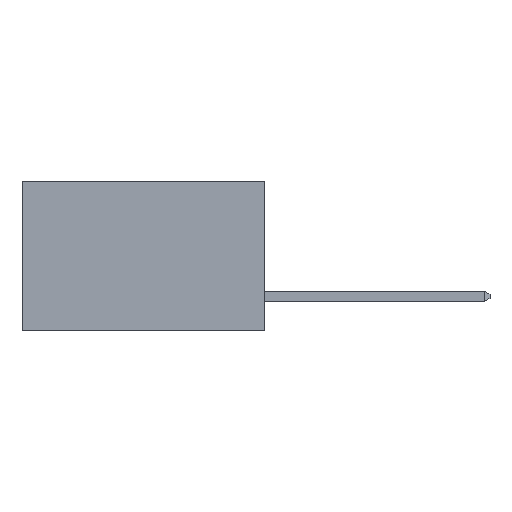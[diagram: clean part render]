
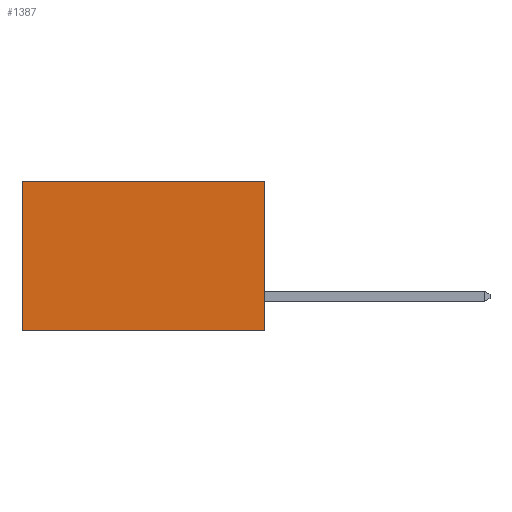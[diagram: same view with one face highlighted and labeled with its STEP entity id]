
A CAD part, left-side view. The second image highlights one B-rep face of the part: STEP entity #1387.
In plain terms, the highlighted planar face has unit normal (-1, 0, 0).
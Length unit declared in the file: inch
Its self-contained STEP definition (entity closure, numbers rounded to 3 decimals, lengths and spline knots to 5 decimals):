
#158 = VERTEX_POINT ( 'NONE', #6100 ) ;
#322 = EDGE_CURVE ( 'NONE', #1749, #3435, #7476, .T. ) ;
#447 = CARTESIAN_POINT ( 'NONE',  ( 0.2615, 0., 0. ) ) ;
#609 = DIRECTION ( 'NONE',  ( 0., 0., -1. ) ) ;
#1137 = VECTOR ( 'NONE', #8581, 39.37008 ) ;
#1387 = ADVANCED_FACE ( 'NONE', ( #3608 ), #4067, .F. ) ;
#1579 = EDGE_CURVE ( 'NONE', #158, #5817, #5837, .T. ) ;
#1749 = VERTEX_POINT ( 'NONE', #447 ) ;
#2723 = LINE ( 'NONE', #9731, #5181 ) ;
#3435 = VERTEX_POINT ( 'NONE', #5038 ) ;
#3608 = FACE_OUTER_BOUND ( 'NONE', #4856, .T. ) ;
#4022 = CARTESIAN_POINT ( 'NONE',  ( 0.2615, 0., 0. ) ) ;
#4067 = PLANE ( 'NONE',  #5044 ) ;
#4185 = ORIENTED_EDGE ( 'NONE', *, *, #1579, .F. ) ;
#4652 = LINE ( 'NONE', #5059, #7953 ) ;
#4720 = EDGE_CURVE ( 'NONE', #1749, #158, #2723, .T. ) ;
#4856 = EDGE_LOOP ( 'NONE', ( #6600, #4185, #8238, #8436 ) ) ;
#5038 = CARTESIAN_POINT ( 'NONE',  ( 0.2615, 0.6, 0. ) ) ;
#5044 = AXIS2_PLACEMENT_3D ( 'NONE', #8011, #8101, #8161 ) ;
#5059 = CARTESIAN_POINT ( 'NONE',  ( 0.2615, 0.6, -0.37 ) ) ;
#5181 = VECTOR ( 'NONE', #9720, 39.37008 ) ;
#5282 = CARTESIAN_POINT ( 'NONE',  ( 0.2615, 0.6, -0.37 ) ) ;
#5381 = VECTOR ( 'NONE', #9350, 39.37008 ) ;
#5817 = VERTEX_POINT ( 'NONE', #5282 ) ;
#5837 = LINE ( 'NONE', #9331, #5381 ) ;
#6100 = CARTESIAN_POINT ( 'NONE',  ( 0.2615, 0., -0.37 ) ) ;
#6600 = ORIENTED_EDGE ( 'NONE', *, *, #8048, .T. ) ;
#7476 = LINE ( 'NONE', #4022, #1137 ) ;
#7953 = VECTOR ( 'NONE', #609, 39.37008 ) ;
#8011 = CARTESIAN_POINT ( 'NONE',  ( 0.2615, 0., -0.37 ) ) ;
#8048 = EDGE_CURVE ( 'NONE', #3435, #5817, #4652, .T. ) ;
#8101 = DIRECTION ( 'NONE',  ( 1., 0., 0. ) ) ;
#8161 = DIRECTION ( 'NONE',  ( 0., 0., -1. ) ) ;
#8238 = ORIENTED_EDGE ( 'NONE', *, *, #4720, .F. ) ;
#8436 = ORIENTED_EDGE ( 'NONE', *, *, #322, .T. ) ;
#8581 = DIRECTION ( 'NONE',  ( 0., 1., 0. ) ) ;
#9331 = CARTESIAN_POINT ( 'NONE',  ( 0.2615, 0., -0.37 ) ) ;
#9350 = DIRECTION ( 'NONE',  ( 0., 1., 0. ) ) ;
#9720 = DIRECTION ( 'NONE',  ( 0., 0., -1. ) ) ;
#9731 = CARTESIAN_POINT ( 'NONE',  ( 0.2615, 0., -0.37 ) ) ;
